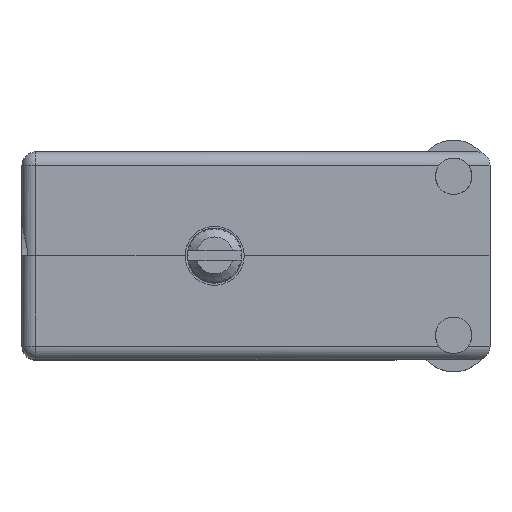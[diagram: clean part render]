
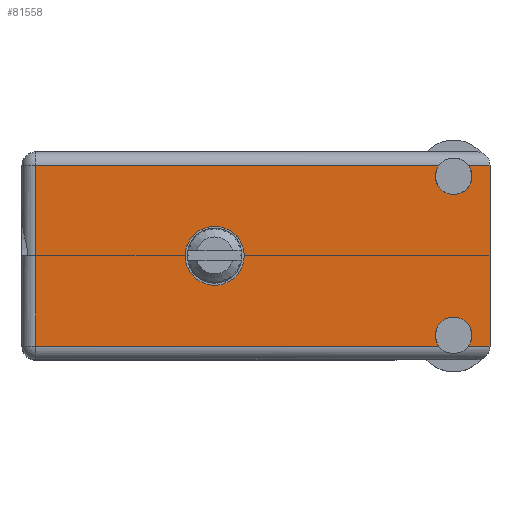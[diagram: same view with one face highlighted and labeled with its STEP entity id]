
A CAD part, top view. The second image highlights one B-rep face of the part: STEP entity #81558.
In plain terms, the highlighted face is planar.
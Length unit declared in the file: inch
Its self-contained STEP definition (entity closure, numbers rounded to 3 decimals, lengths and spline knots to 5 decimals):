
#1737 = CARTESIAN_POINT ( 'NONE',  ( 0., 0.806, -0.1015 ) ) ;
#2589 = AXIS2_PLACEMENT_3D ( 'NONE', #166601, #28218, #29222 ) ;
#3301 = CARTESIAN_POINT ( 'NONE',  ( -0.6625, 0.806, -0.3575 ) ) ;
#4263 = DIRECTION ( 'NONE',  ( 0., 0., 1. ) ) ;
#8504 = ORIENTED_EDGE ( 'NONE', *, *, #140958, .F. ) ;
#8926 = CARTESIAN_POINT ( 'NONE',  ( 0., 0.806, 0. ) ) ;
#9043 = CARTESIAN_POINT ( 'NONE',  ( 0.8215, 0.806, 0.211 ) ) ;
#14482 = EDGE_CURVE ( 'NONE', #34229, #172346, #92178, .T. ) ;
#14827 = ORIENTED_EDGE ( 'NONE', *, *, #14482, .F. ) ;
#18032 = EDGE_CURVE ( 'NONE', #106367, #70970, #181573, .T. ) ;
#18066 = AXIS2_PLACEMENT_3D ( 'NONE', #8926, #57366, #4263 ) ;
#18792 = CARTESIAN_POINT ( 'NONE',  ( 0., 0.806, 0.1015 ) ) ;
#20203 = CARTESIAN_POINT ( 'NONE',  ( 0.8215, 0.806, 0.2735 ) ) ;
#23093 = LINE ( 'NONE', #82706, #149653 ) ;
#25134 = CARTESIAN_POINT ( 'NONE',  ( -0.6155, 0.806, -0.3575 ) ) ;
#26117 = DIRECTION ( 'NONE',  ( 0., 0., 1. ) ) ;
#26955 = CARTESIAN_POINT ( 'NONE',  ( 0.8215, 0.806, 0.2735 ) ) ;
#28065 = VECTOR ( 'NONE', #49547, 39.37008 ) ;
#28218 = DIRECTION ( 'NONE',  ( 0., 1., 0. ) ) ;
#29222 = DIRECTION ( 'NONE',  ( 0., 0., 1. ) ) ;
#30407 = AXIS2_PLACEMENT_3D ( 'NONE', #26955, #196604, #91558 ) ;
#33862 = CARTESIAN_POINT ( 'NONE',  ( 0., 0.806, 0. ) ) ;
#34229 = VERTEX_POINT ( 'NONE', #1737 ) ;
#35130 = AXIS2_PLACEMENT_3D ( 'NONE', #20203, #143428, #111120 ) ;
#37527 = DIRECTION ( 'NONE',  ( -1., 0., 0. ) ) ;
#39242 = EDGE_LOOP ( 'NONE', ( #86400, #57118, #133710, #110519, #141181, #155980, #66498, #8504, #110357, #65548 ) ) ;
#40910 = EDGE_CURVE ( 'NONE', #155516, #153734, #23093, .T. ) ;
#41320 = CIRCLE ( 'NONE', #2589, 0.0625 ) ;
#42036 = CARTESIAN_POINT ( 'NONE',  ( 0.9465, 0.806, -0.3105 ) ) ;
#44057 = CARTESIAN_POINT ( 'NONE',  ( 0.8215, 0.806, -0.211 ) ) ;
#49547 = DIRECTION ( 'NONE',  ( 1., 0., 0. ) ) ;
#50303 = EDGE_CURVE ( 'NONE', #70970, #182558, #92294, .T. ) ;
#53649 = DIRECTION ( 'NONE',  ( 0., 1., 0. ) ) ;
#57118 = ORIENTED_EDGE ( 'NONE', *, *, #152209, .F. ) ;
#57366 = DIRECTION ( 'NONE',  ( 0., 1., 0. ) ) ;
#59001 = DIRECTION ( 'NONE',  ( 1., 0., 0. ) ) ;
#61684 = CARTESIAN_POINT ( 'NONE',  ( 0.77113, 0.806, 0.3105 ) ) ;
#62983 = CARTESIAN_POINT ( 'NONE',  ( -0.6625, 0.806, -0.3105 ) ) ;
#65548 = ORIENTED_EDGE ( 'NONE', *, *, #18032, .T. ) ;
#65865 = FACE_BOUND ( 'NONE', #104829, .T. ) ;
#66498 = ORIENTED_EDGE ( 'NONE', *, *, #103629, .F. ) ;
#70970 = VERTEX_POINT ( 'NONE', #100923 ) ;
#72408 = AXIS2_PLACEMENT_3D ( 'NONE', #152653, #88019, #151664 ) ;
#75974 = AXIS2_PLACEMENT_3D ( 'NONE', #3301, #53649, #37527 ) ;
#78443 = CARTESIAN_POINT ( 'NONE',  ( 0.77113, 0.806, -0.3105 ) ) ;
#80882 = LINE ( 'NONE', #156653, #28065 ) ;
#81558 = ADVANCED_FACE ( 'NONE', ( #65865, #126465 ), #83988, .T. ) ;
#82706 = CARTESIAN_POINT ( 'NONE',  ( 0.9465, 0.806, 0.3575 ) ) ;
#82869 = VECTOR ( 'NONE', #172060, 39.37008 ) ;
#83988 = PLANE ( 'NONE',  #75974 ) ;
#86400 = ORIENTED_EDGE ( 'NONE', *, *, #50303, .T. ) ;
#88019 = DIRECTION ( 'NONE',  ( 0., 1., 0. ) ) ;
#89138 = VECTOR ( 'NONE', #26117, 39.37008 ) ;
#89205 = CARTESIAN_POINT ( 'NONE',  ( 0.87187, 0.806, -0.3105 ) ) ;
#89528 = EDGE_CURVE ( 'NONE', #133341, #106367, #199356, .T. ) ;
#90510 = ORIENTED_EDGE ( 'NONE', *, *, #178988, .F. ) ;
#91558 = DIRECTION ( 'NONE',  ( 0., 0., 1. ) ) ;
#92178 = CIRCLE ( 'NONE', #18066, 0.1015 ) ;
#92294 = LINE ( 'NONE', #104446, #154437 ) ;
#98857 = EDGE_CURVE ( 'NONE', #173773, #153734, #80882, .T. ) ;
#100923 = CARTESIAN_POINT ( 'NONE',  ( -0.6155, 0.806, 0.3105 ) ) ;
#103629 = EDGE_CURVE ( 'NONE', #169657, #106787, #41320, .T. ) ;
#104446 = CARTESIAN_POINT ( 'NONE',  ( 0.9465, 0.806, 0.3105 ) ) ;
#104829 = EDGE_LOOP ( 'NONE', ( #90510, #14827 ) ) ;
#106367 = VERTEX_POINT ( 'NONE', #136386 ) ;
#106787 = VERTEX_POINT ( 'NONE', #89205 ) ;
#110357 = ORIENTED_EDGE ( 'NONE', *, *, #89528, .T. ) ;
#110519 = ORIENTED_EDGE ( 'NONE', *, *, #98857, .T. ) ;
#111120 = DIRECTION ( 'NONE',  ( 0., 0., 1. ) ) ;
#117432 = CIRCLE ( 'NONE', #30407, 0.0625 ) ;
#124014 = CIRCLE ( 'NONE', #72408, 0.0625 ) ;
#126465 = FACE_OUTER_BOUND ( 'NONE', #39242, .T. ) ;
#129369 = CARTESIAN_POINT ( 'NONE',  ( 0.9465, 0.806, 0.3105 ) ) ;
#133272 = VECTOR ( 'NONE', #161064, 39.37008 ) ;
#133341 = VERTEX_POINT ( 'NONE', #78443 ) ;
#133710 = ORIENTED_EDGE ( 'NONE', *, *, #182680, .F. ) ;
#134870 = AXIS2_PLACEMENT_3D ( 'NONE', #33862, #183372, #199524 ) ;
#135313 = EDGE_CURVE ( 'NONE', #155516, #106787, #160069, .T. ) ;
#136352 = CARTESIAN_POINT ( 'NONE',  ( 0.87187, 0.806, 0.3105 ) ) ;
#136386 = CARTESIAN_POINT ( 'NONE',  ( -0.6155, 0.806, -0.3105 ) ) ;
#140958 = EDGE_CURVE ( 'NONE', #133341, #169657, #124014, .T. ) ;
#141181 = ORIENTED_EDGE ( 'NONE', *, *, #40910, .F. ) ;
#143428 = DIRECTION ( 'NONE',  ( 0., 1., 0. ) ) ;
#144829 = CIRCLE ( 'NONE', #35130, 0.0625 ) ;
#149653 = VECTOR ( 'NONE', #188759, 39.37008 ) ;
#151664 = DIRECTION ( 'NONE',  ( 0., 0., 1. ) ) ;
#152209 = EDGE_CURVE ( 'NONE', #164973, #182558, #117432, .T. ) ;
#152653 = CARTESIAN_POINT ( 'NONE',  ( 0.8215, 0.806, -0.2735 ) ) ;
#153734 = VERTEX_POINT ( 'NONE', #129369 ) ;
#154239 = CIRCLE ( 'NONE', #134870, 0.1015 ) ;
#154437 = VECTOR ( 'NONE', #59001, 39.37008 ) ;
#155516 = VERTEX_POINT ( 'NONE', #42036 ) ;
#155980 = ORIENTED_EDGE ( 'NONE', *, *, #135313, .T. ) ;
#156653 = CARTESIAN_POINT ( 'NONE',  ( 0.9465, 0.806, 0.3105 ) ) ;
#160069 = LINE ( 'NONE', #194302, #133272 ) ;
#161064 = DIRECTION ( 'NONE',  ( -1., 0., 0. ) ) ;
#164973 = VERTEX_POINT ( 'NONE', #9043 ) ;
#166601 = CARTESIAN_POINT ( 'NONE',  ( 0.8215, 0.806, -0.2735 ) ) ;
#169657 = VERTEX_POINT ( 'NONE', #44057 ) ;
#172060 = DIRECTION ( 'NONE',  ( -1., 0., 0. ) ) ;
#172346 = VERTEX_POINT ( 'NONE', #18792 ) ;
#173773 = VERTEX_POINT ( 'NONE', #136352 ) ;
#178988 = EDGE_CURVE ( 'NONE', #172346, #34229, #154239, .T. ) ;
#181573 = LINE ( 'NONE', #25134, #89138 ) ;
#182558 = VERTEX_POINT ( 'NONE', #61684 ) ;
#182680 = EDGE_CURVE ( 'NONE', #173773, #164973, #144829, .T. ) ;
#183372 = DIRECTION ( 'NONE',  ( 0., 1., 0. ) ) ;
#188759 = DIRECTION ( 'NONE',  ( 0., 0., 1. ) ) ;
#194302 = CARTESIAN_POINT ( 'NONE',  ( -0.6625, 0.806, -0.3105 ) ) ;
#196604 = DIRECTION ( 'NONE',  ( 0., 1., 0. ) ) ;
#199356 = LINE ( 'NONE', #62983, #82869 ) ;
#199524 = DIRECTION ( 'NONE',  ( 0., 0., 1. ) ) ;
